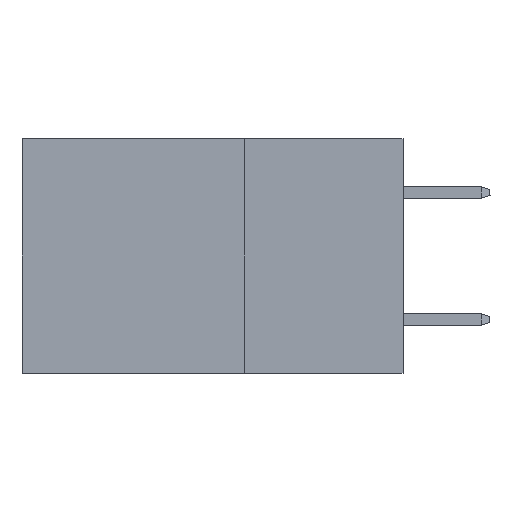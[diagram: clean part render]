
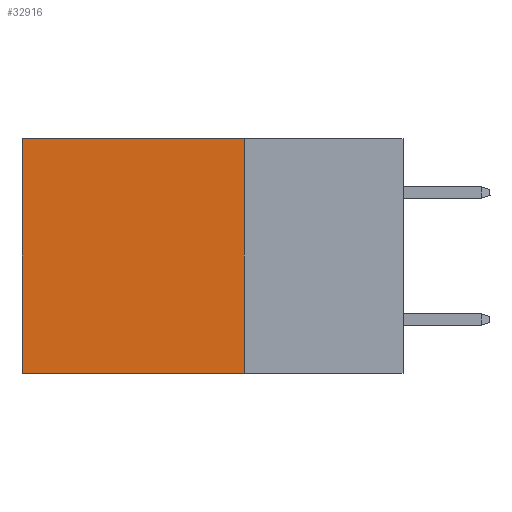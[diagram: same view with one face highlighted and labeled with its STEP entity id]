
A CAD part, left-side view. The second image highlights one B-rep face of the part: STEP entity #32916.
In plain terms, the highlighted planar face has unit normal (-1, 0, 0).
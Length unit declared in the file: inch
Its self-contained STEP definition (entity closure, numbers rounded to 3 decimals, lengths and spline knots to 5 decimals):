
#838 = CARTESIAN_POINT ( 'NONE',  ( 0.2875, 0.25, -0.37 ) ) ;
#6646 = VECTOR ( 'NONE', #45879, 39.37008 ) ;
#6905 = EDGE_CURVE ( 'NONE', #40675, #27217, #7777, .T. ) ;
#7329 = ORIENTED_EDGE ( 'NONE', *, *, #38001, .T. ) ;
#7777 = LINE ( 'NONE', #12485, #45114 ) ;
#9707 = CARTESIAN_POINT ( 'NONE',  ( 0.2875, 0.6, 0. ) ) ;
#12485 = CARTESIAN_POINT ( 'NONE',  ( 0.2875, 0.25, 0. ) ) ;
#13367 = CARTESIAN_POINT ( 'NONE',  ( 0.2875, 0.25, 0. ) ) ;
#13998 = CARTESIAN_POINT ( 'NONE',  ( 0.2875, 0.25, 0. ) ) ;
#15545 = ORIENTED_EDGE ( 'NONE', *, *, #36288, .T. ) ;
#16219 = EDGE_LOOP ( 'NONE', ( #7329, #28015, #20585, #15545 ) ) ;
#17332 = LINE ( 'NONE', #17568, #6646 ) ;
#17568 = CARTESIAN_POINT ( 'NONE',  ( 0.2875, 0.25, -0.37 ) ) ;
#20585 = ORIENTED_EDGE ( 'NONE', *, *, #6905, .F. ) ;
#20858 = LINE ( 'NONE', #13998, #27663 ) ;
#21574 = CARTESIAN_POINT ( 'NONE',  ( 0.2875, 0.25, 0. ) ) ;
#22277 = AXIS2_PLACEMENT_3D ( 'NONE', #21574, #28887, #38777 ) ;
#24418 = VERTEX_POINT ( 'NONE', #35742 ) ;
#27217 = VERTEX_POINT ( 'NONE', #838 ) ;
#27663 = VECTOR ( 'NONE', #35217, 39.37008 ) ;
#28015 = ORIENTED_EDGE ( 'NONE', *, *, #45607, .F. ) ;
#28887 = DIRECTION ( 'NONE',  ( 1., 0., 0. ) ) ;
#31708 = PLANE ( 'NONE',  #22277 ) ;
#31877 = LINE ( 'NONE', #9707, #44349 ) ;
#32916 = ADVANCED_FACE ( 'NONE', ( #35708 ), #31708, .F. ) ;
#33642 = VERTEX_POINT ( 'NONE', #45686 ) ;
#35217 = DIRECTION ( 'NONE',  ( 0., 1., 0. ) ) ;
#35708 = FACE_OUTER_BOUND ( 'NONE', #16219, .T. ) ;
#35742 = CARTESIAN_POINT ( 'NONE',  ( 0.2875, 0.6, 0. ) ) ;
#36288 = EDGE_CURVE ( 'NONE', #40675, #24418, #20858, .T. ) ;
#36780 = DIRECTION ( 'NONE',  ( 0., 0., -1. ) ) ;
#38001 = EDGE_CURVE ( 'NONE', #24418, #33642, #31877, .T. ) ;
#38777 = DIRECTION ( 'NONE',  ( 0., 0., -1. ) ) ;
#38949 = DIRECTION ( 'NONE',  ( 0., 0., -1. ) ) ;
#40675 = VERTEX_POINT ( 'NONE', #13367 ) ;
#44349 = VECTOR ( 'NONE', #38949, 39.37008 ) ;
#45114 = VECTOR ( 'NONE', #36780, 39.37008 ) ;
#45607 = EDGE_CURVE ( 'NONE', #27217, #33642, #17332, .T. ) ;
#45686 = CARTESIAN_POINT ( 'NONE',  ( 0.2875, 0.6, -0.37 ) ) ;
#45879 = DIRECTION ( 'NONE',  ( 0., 1., 0. ) ) ;
